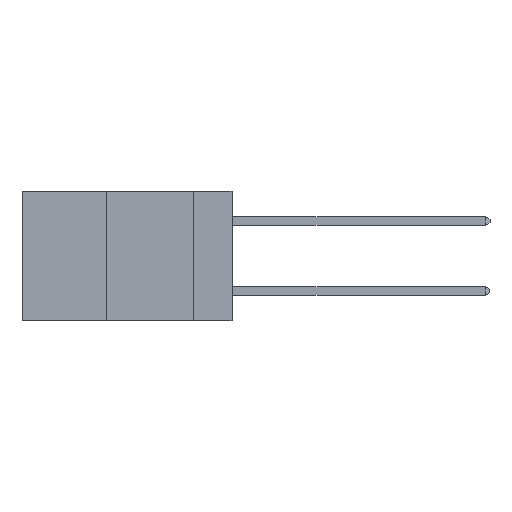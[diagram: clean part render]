
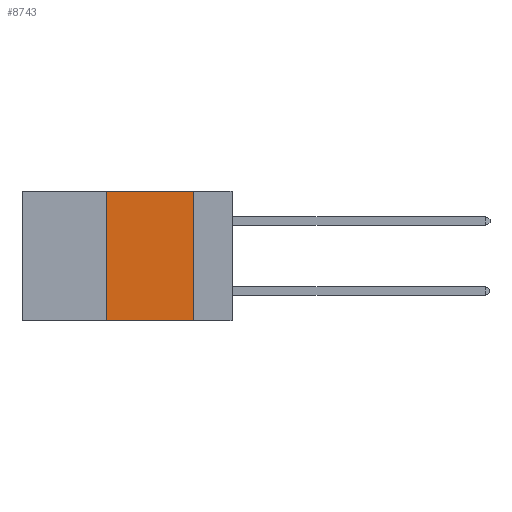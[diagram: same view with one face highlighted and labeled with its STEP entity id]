
A CAD part, left-side view. The second image highlights one B-rep face of the part: STEP entity #8743.
In plain terms, the highlighted planar face has unit normal (-1, 0, 0).
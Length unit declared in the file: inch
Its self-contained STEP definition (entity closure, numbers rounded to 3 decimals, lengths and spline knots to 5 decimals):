
#710 = DIRECTION ( 'NONE',  ( 0., 0., -1. ) ) ;
#1476 = ORIENTED_EDGE ( 'NONE', *, *, #4459, .F. ) ;
#2454 = CARTESIAN_POINT ( 'NONE',  ( 0., 0.11, 0. ) ) ;
#2813 = CARTESIAN_POINT ( 'NONE',  ( 0., 0.36, 0. ) ) ;
#3181 = EDGE_CURVE ( 'NONE', #17373, #10115, #8536, .T. ) ;
#4459 = EDGE_CURVE ( 'NONE', #19034, #22438, #21770, .T. ) ;
#4678 = DIRECTION ( 'NONE',  ( 0., 0., 1. ) ) ;
#4851 = EDGE_LOOP ( 'NONE', ( #1476, #16157, #19481, #9388 ) ) ;
#4919 = CARTESIAN_POINT ( 'NONE',  ( 0., 0.11, -0.37 ) ) ;
#6480 = AXIS2_PLACEMENT_3D ( 'NONE', #19074, #11831, #710 ) ;
#6895 = CARTESIAN_POINT ( 'NONE',  ( 0., 0.6, 0. ) ) ;
#7203 = VECTOR ( 'NONE', #19862, 39.37008 ) ;
#7977 = VECTOR ( 'NONE', #4678, 39.37008 ) ;
#8127 = LINE ( 'NONE', #6895, #21511 ) ;
#8358 = VECTOR ( 'NONE', #18996, 39.37008 ) ;
#8536 = LINE ( 'NONE', #2813, #7977 ) ;
#8743 = ADVANCED_FACE ( 'NONE', ( #12478 ), #15397, .F. ) ;
#8773 = DIRECTION ( 'NONE',  ( 0., -1., 0. ) ) ;
#9388 = ORIENTED_EDGE ( 'NONE', *, *, #20953, .T. ) ;
#10115 = VERTEX_POINT ( 'NONE', #19251 ) ;
#11831 = DIRECTION ( 'NONE',  ( 1., 0., 0. ) ) ;
#12478 = FACE_OUTER_BOUND ( 'NONE', #4851, .T. ) ;
#12629 = CARTESIAN_POINT ( 'NONE',  ( 0., 0.11, 0. ) ) ;
#15397 = PLANE ( 'NONE',  #6480 ) ;
#16157 = ORIENTED_EDGE ( 'NONE', *, *, #19916, .F. ) ;
#17193 = CARTESIAN_POINT ( 'NONE',  ( 0., 0.6, -0.37 ) ) ;
#17373 = VERTEX_POINT ( 'NONE', #23202 ) ;
#18108 = LINE ( 'NONE', #17193, #8358 ) ;
#18996 = DIRECTION ( 'NONE',  ( 0., -1., 0. ) ) ;
#19034 = VERTEX_POINT ( 'NONE', #2454 ) ;
#19074 = CARTESIAN_POINT ( 'NONE',  ( 0., 0.6, 0. ) ) ;
#19251 = CARTESIAN_POINT ( 'NONE',  ( 0., 0.36, 0. ) ) ;
#19481 = ORIENTED_EDGE ( 'NONE', *, *, #3181, .F. ) ;
#19862 = DIRECTION ( 'NONE',  ( 0., 0., -1. ) ) ;
#19916 = EDGE_CURVE ( 'NONE', #10115, #19034, #8127, .T. ) ;
#20953 = EDGE_CURVE ( 'NONE', #17373, #22438, #18108, .T. ) ;
#21511 = VECTOR ( 'NONE', #8773, 39.37008 ) ;
#21770 = LINE ( 'NONE', #12629, #7203 ) ;
#22438 = VERTEX_POINT ( 'NONE', #4919 ) ;
#23202 = CARTESIAN_POINT ( 'NONE',  ( 0., 0.36, -0.37 ) ) ;
